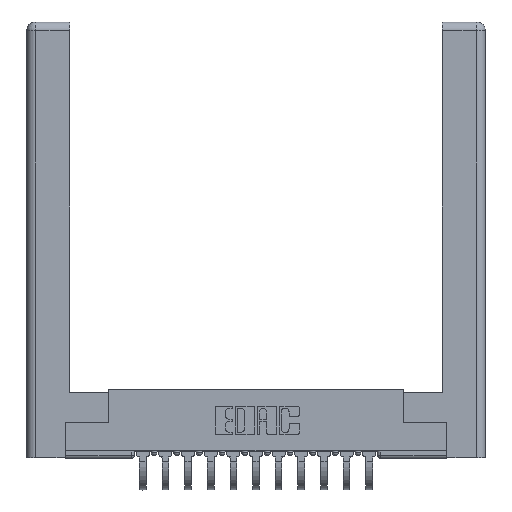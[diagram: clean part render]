
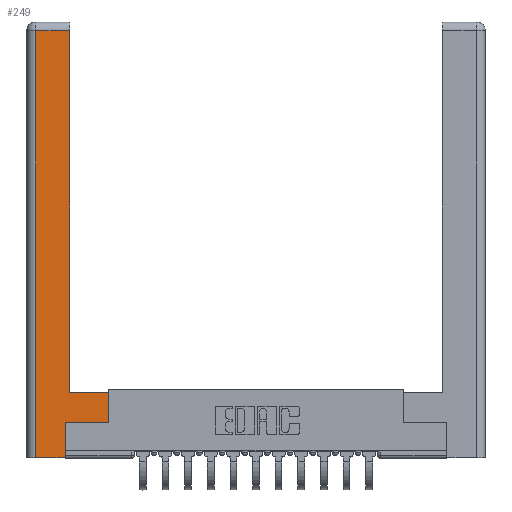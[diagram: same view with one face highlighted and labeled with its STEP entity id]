
A CAD part, top view. The second image highlights one B-rep face of the part: STEP entity #249.
In plain terms, the highlighted planar face has unit normal (0, 0, 1).
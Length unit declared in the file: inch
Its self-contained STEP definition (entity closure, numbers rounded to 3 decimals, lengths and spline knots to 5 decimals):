
#184 = ORIENTED_EDGE ( 'NONE', *, *, #15906, .T. ) ;
#249 = ADVANCED_FACE ( 'NONE', ( #14730 ), #3655, .F. ) ;
#365 = ORIENTED_EDGE ( 'NONE', *, *, #16059, .T. ) ;
#658 = VERTEX_POINT ( 'NONE', #13255 ) ;
#937 = VERTEX_POINT ( 'NONE', #6112 ) ;
#1028 = CARTESIAN_POINT ( 'NONE',  ( 0.565, 0.245, 0. ) ) ;
#1144 = CARTESIAN_POINT ( 'NONE',  ( 0.265, 0., 0. ) ) ;
#1173 = VECTOR ( 'NONE', #12771, 39.37008 ) ;
#1416 = VECTOR ( 'NONE', #6737, 39.37008 ) ;
#1428 = VECTOR ( 'NONE', #2999, 39.37008 ) ;
#1707 = EDGE_CURVE ( 'NONE', #10785, #16454, #10151, .T. ) ;
#2442 = DIRECTION ( 'NONE',  ( 0., -1., 0. ) ) ;
#2874 = VECTOR ( 'NONE', #2442, 39.37008 ) ;
#2999 = DIRECTION ( 'NONE',  ( 0., 1., 0. ) ) ;
#3204 = EDGE_CURVE ( 'NONE', #7784, #3253, #5765, .T. ) ;
#3253 = VERTEX_POINT ( 'NONE', #16588 ) ;
#3655 = PLANE ( 'NONE',  #8228 ) ;
#3882 = CARTESIAN_POINT ( 'NONE',  ( 0.295, 2.94, 0. ) ) ;
#3966 = EDGE_CURVE ( 'NONE', #9669, #658, #10539, .T. ) ;
#4206 = ORIENTED_EDGE ( 'NONE', *, *, #3966, .T. ) ;
#5106 = LINE ( 'NONE', #1028, #17011 ) ;
#5138 = ORIENTED_EDGE ( 'NONE', *, *, #1707, .T. ) ;
#5178 = EDGE_CURVE ( 'NONE', #16454, #12826, #11786, .T. ) ;
#5765 = LINE ( 'NONE', #12360, #1428 ) ;
#5793 = DIRECTION ( 'NONE',  ( 0., 1., 0. ) ) ;
#5900 = VECTOR ( 'NONE', #16195, 39.37008 ) ;
#6112 = CARTESIAN_POINT ( 'NONE',  ( 0.265, 0.245, 0. ) ) ;
#6737 = DIRECTION ( 'NONE',  ( 1., 0., 0. ) ) ;
#7289 = LINE ( 'NONE', #11545, #13118 ) ;
#7784 = VERTEX_POINT ( 'NONE', #11406 ) ;
#8024 = DIRECTION ( 'NONE',  ( 0., 0., -1. ) ) ;
#8228 = AXIS2_PLACEMENT_3D ( 'NONE', #11929, #8024, #11834 ) ;
#9044 = EDGE_CURVE ( 'NONE', #658, #937, #10991, .T. ) ;
#9669 = VERTEX_POINT ( 'NONE', #15796 ) ;
#9773 = ORIENTED_EDGE ( 'NONE', *, *, #10202, .T. ) ;
#9793 = CARTESIAN_POINT ( 'NONE',  ( 0.295, 0.45, 0. ) ) ;
#10151 = LINE ( 'NONE', #16792, #13642 ) ;
#10202 = EDGE_CURVE ( 'NONE', #937, #7784, #5106, .T. ) ;
#10449 = CARTESIAN_POINT ( 'NONE',  ( 0.0615, 2.94, 0. ) ) ;
#10539 = LINE ( 'NONE', #1144, #1416 ) ;
#10785 = VERTEX_POINT ( 'NONE', #9793 ) ;
#10914 = EDGE_LOOP ( 'NONE', ( #5138, #16105, #365, #4206, #14669, #9773, #17415, #184 ) ) ;
#10991 = LINE ( 'NONE', #12321, #5900 ) ;
#11406 = CARTESIAN_POINT ( 'NONE',  ( 0.565, 0.245, 0. ) ) ;
#11545 = CARTESIAN_POINT ( 'NONE',  ( 0.295, 0.45, 0. ) ) ;
#11786 = LINE ( 'NONE', #10449, #1173 ) ;
#11834 = DIRECTION ( 'NONE',  ( -1., 0., 0. ) ) ;
#11929 = CARTESIAN_POINT ( 'NONE',  ( 0., 0., 0. ) ) ;
#12321 = CARTESIAN_POINT ( 'NONE',  ( 0.265, 0.245, 0. ) ) ;
#12360 = CARTESIAN_POINT ( 'NONE',  ( 0.565, 0.45, 0. ) ) ;
#12771 = DIRECTION ( 'NONE',  ( -1., 0., 0. ) ) ;
#12826 = VERTEX_POINT ( 'NONE', #13234 ) ;
#13118 = VECTOR ( 'NONE', #17035, 39.37008 ) ;
#13234 = CARTESIAN_POINT ( 'NONE',  ( 0.0615, 2.94, 0. ) ) ;
#13255 = CARTESIAN_POINT ( 'NONE',  ( 0.265, 0., 0. ) ) ;
#13642 = VECTOR ( 'NONE', #5793, 39.37008 ) ;
#14656 = DIRECTION ( 'NONE',  ( 1., 0., 0. ) ) ;
#14669 = ORIENTED_EDGE ( 'NONE', *, *, #9044, .T. ) ;
#14701 = CARTESIAN_POINT ( 'NONE',  ( 0.0615, 0., 0. ) ) ;
#14730 = FACE_OUTER_BOUND ( 'NONE', #10914, .T. ) ;
#15796 = CARTESIAN_POINT ( 'NONE',  ( 0.0615, 0., 0. ) ) ;
#15906 = EDGE_CURVE ( 'NONE', #3253, #10785, #7289, .T. ) ;
#16046 = LINE ( 'NONE', #14701, #2874 ) ;
#16059 = EDGE_CURVE ( 'NONE', #12826, #9669, #16046, .T. ) ;
#16105 = ORIENTED_EDGE ( 'NONE', *, *, #5178, .T. ) ;
#16195 = DIRECTION ( 'NONE',  ( 0., 1., 0. ) ) ;
#16454 = VERTEX_POINT ( 'NONE', #3882 ) ;
#16588 = CARTESIAN_POINT ( 'NONE',  ( 0.565, 0.45, 0. ) ) ;
#16792 = CARTESIAN_POINT ( 'NONE',  ( 0.295, 3., 0. ) ) ;
#17011 = VECTOR ( 'NONE', #14656, 39.37008 ) ;
#17035 = DIRECTION ( 'NONE',  ( -1., 0., 0. ) ) ;
#17415 = ORIENTED_EDGE ( 'NONE', *, *, #3204, .T. ) ;
